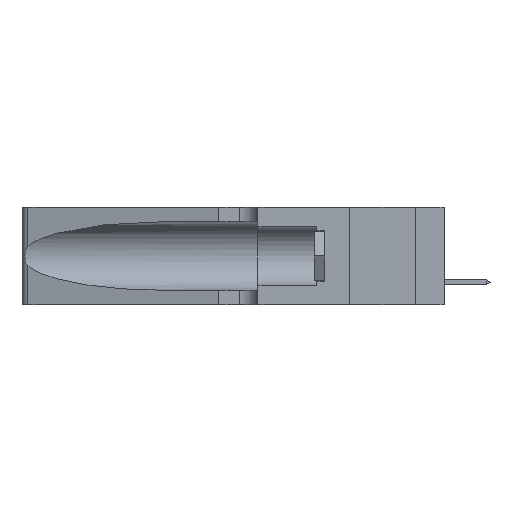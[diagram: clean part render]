
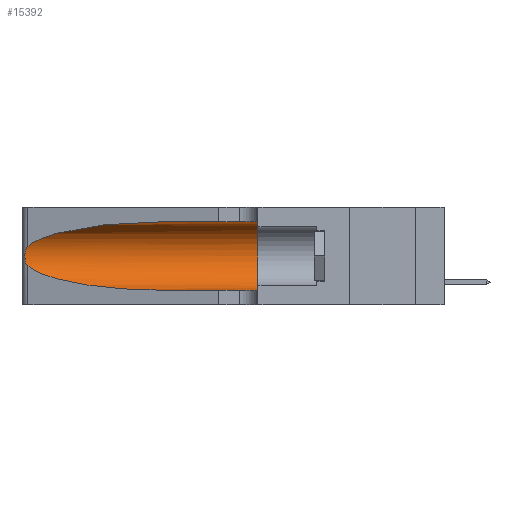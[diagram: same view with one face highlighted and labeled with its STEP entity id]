
A CAD part, left-side view. The second image highlights one B-rep face of the part: STEP entity #15392.
In plain terms, the highlighted cylindrical face has radius 3.308 mm (diameter 6.617 mm), a partial arc.
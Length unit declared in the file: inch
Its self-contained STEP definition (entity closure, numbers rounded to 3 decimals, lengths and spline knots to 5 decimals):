
#442 = EDGE_CURVE ( 'NONE', #17372, #2219, #3135, .T. ) ;
#567 = CARTESIAN_POINT ( 'NONE',  ( 0.26017, 1.23833, 0.17102 ) ) ;
#684 = DIRECTION ( 'NONE',  ( 0., -1., 0. ) ) ;
#1169 = LINE ( 'NONE', #15823, #13541 ) ;
#1185 = DIRECTION ( 'NONE',  ( 0., 1., 0. ) ) ;
#1220 = EDGE_CURVE ( 'NONE', #7691, #2219, #16147, .T. ) ;
#1266 = DIRECTION ( 'NONE',  ( 0., 0., -1. ) ) ;
#1465 = CARTESIAN_POINT ( 'NONE',  ( 0.18966, 0.96281, 0.05475 ) ) ;
#1614 = EDGE_CURVE ( 'NONE', #13062, #11561, #14338, .T. ) ;
#1767 = ORIENTED_EDGE ( 'NONE', *, *, #1220, .T. ) ;
#2219 = VERTEX_POINT ( 'NONE', #5747 ) ;
#2413 = CARTESIAN_POINT ( 'NONE',  ( 0.1305, 0.72297, 0.05475 ) ) ;
#2614 = CARTESIAN_POINT ( 'NONE',  ( 0.1305, 0.35, 0.185 ) ) ;
#3135 = CIRCLE ( 'NONE', #15075, 0.13025 ) ;
#3391 = CARTESIAN_POINT ( 'NONE',  ( 0.26075, 1.23896, 0.19203 ) ) ;
#3633 = CARTESIAN_POINT ( 'NONE',  ( 0.1305, 0.72297, 0.05475 ) ) ;
#4206 = CARTESIAN_POINT ( 'NONE',  ( 0.25487, 1.22718, 0.14631 ) ) ;
#4277 = CARTESIAN_POINT ( 'NONE',  ( 0.1305, 0.72297, 0.31525 ) ) ;
#4448 =( BOUNDED_CURVE ( )  B_SPLINE_CURVE ( 3, ( #14087, #8386, #5746, #15411 ),
 .UNSPECIFIED., .F., .F. ) 
 B_SPLINE_CURVE_WITH_KNOTS ( ( 4, 4 ),
 ( 1.5708, 2.84003 ),
 .UNSPECIFIED. ) 
 CURVE ( )  GEOMETRIC_REPRESENTATION_ITEM ( )  RATIONAL_B_SPLINE_CURVE ( ( 1., 0.87, 0.87, 1. ) ) 
 REPRESENTATION_ITEM ( '' )  );
#4646 = EDGE_CURVE ( 'NONE', #10492, #13062, #4448, .T. ) ;
#4760 = CARTESIAN_POINT ( 'NONE',  ( 0.25487, 1.22718, 0.14631 ) ) ;
#4889 = ORIENTED_EDGE ( 'NONE', *, *, #1614, .T. ) ;
#4906 = CARTESIAN_POINT ( 'NONE',  ( 0.25555, 1.22994, 0.2215 ) ) ;
#5062 = VECTOR ( 'NONE', #5111, 39.37008 ) ;
#5111 = DIRECTION ( 'NONE',  ( 0., -1., 0. ) ) ;
#5331 = DIRECTION ( 'NONE',  ( 0., -1., 0. ) ) ;
#5746 = CARTESIAN_POINT ( 'NONE',  ( 0.2373, 1.15595, 0.28018 ) ) ;
#5747 = CARTESIAN_POINT ( 'NONE',  ( 0.1305, 0.35, 0.05475 ) ) ;
#5951 = EDGE_LOOP ( 'NONE', ( #15759, #4889, #10830, #1767, #12517, #6734 ) ) ;
#6129 = CARTESIAN_POINT ( 'NONE',  ( 0.25856, 1.23593, 0.16098 ) ) ;
#6188 = CARTESIAN_POINT ( 'NONE',  ( 0.26075, 1.23896, 0.178 ) ) ;
#6292 = CARTESIAN_POINT ( 'NONE',  ( 0.25555, 1.22993, 0.14849 ) ) ;
#6547 =( BOUNDED_CURVE ( )  B_SPLINE_CURVE ( 3, ( #4206, #6991, #1465, #2413 ),
 .UNSPECIFIED., .F., .F. ) 
 B_SPLINE_CURVE_WITH_KNOTS ( ( 4, 4 ),
 ( 3.44316, 4.71239 ),
 .UNSPECIFIED. ) 
 CURVE ( )  GEOMETRIC_REPRESENTATION_ITEM ( )  RATIONAL_B_SPLINE_CURVE ( ( 1., 0.87, 0.87, 1. ) ) 
 REPRESENTATION_ITEM ( '' )  );
#6734 = ORIENTED_EDGE ( 'NONE', *, *, #15949, .F. ) ;
#6991 = CARTESIAN_POINT ( 'NONE',  ( 0.2373, 1.15595, 0.08982 ) ) ;
#7266 = FACE_OUTER_BOUND ( 'NONE', #5951, .T. ) ;
#7455 = CARTESIAN_POINT ( 'NONE',  ( 0.25854, 1.2359, 0.20912 ) ) ;
#7691 = VERTEX_POINT ( 'NONE', #3633 ) ;
#8386 = CARTESIAN_POINT ( 'NONE',  ( 0.18966, 0.96281, 0.31525 ) ) ;
#8954 = CARTESIAN_POINT ( 'NONE',  ( 0.25789, 1.23486, 0.15765 ) ) ;
#9500 = DIRECTION ( 'NONE',  ( 0., 0., 1. ) ) ;
#9523 = CARTESIAN_POINT ( 'NONE',  ( 0.1305, 1.61858, 0.185 ) ) ;
#10270 = CYLINDRICAL_SURFACE ( 'NONE', #12976, 0.13025 ) ;
#10342 = CARTESIAN_POINT ( 'NONE',  ( 0.25639, 1.23186, 0.15144 ) ) ;
#10396 = CARTESIAN_POINT ( 'NONE',  ( 0.25487, 1.22718, 0.22369 ) ) ;
#10492 = VERTEX_POINT ( 'NONE', #4277 ) ;
#10830 = ORIENTED_EDGE ( 'NONE', *, *, #15710, .T. ) ;
#11561 = VERTEX_POINT ( 'NONE', #4760 ) ;
#11693 = CARTESIAN_POINT ( 'NONE',  ( 0.25639, 1.23184, 0.21858 ) ) ;
#12120 = CARTESIAN_POINT ( 'NONE',  ( 0.25487, 1.22718, 0.22369 ) ) ;
#12517 = ORIENTED_EDGE ( 'NONE', *, *, #442, .F. ) ;
#12976 = AXIS2_PLACEMENT_3D ( 'NONE', #9523, #5331, #1266 ) ;
#13062 = VERTEX_POINT ( 'NONE', #12120 ) ;
#13063 = CARTESIAN_POINT ( 'NONE',  ( 0.25787, 1.23484, 0.2124 ) ) ;
#13541 = VECTOR ( 'NONE', #684, 39.37008 ) ;
#14087 = CARTESIAN_POINT ( 'NONE',  ( 0.1305, 0.72297, 0.31525 ) ) ;
#14338 = B_SPLINE_CURVE_WITH_KNOTS ( 'NONE', 3,
 ( #10396, #4906, #11693, #13063, #7455, #14602, #3391, #6188, #567, #6129, #8954, #10342, #6292, #15995 ),
 .UNSPECIFIED., .F., .F.,
 ( 4, 2, 2, 2, 2, 2, 4 ),
 ( 0., 0.00027, 0.00053, 0.00107, 0.0016, 0.00187, 0.00214 ),
 .UNSPECIFIED. ) ;
#14398 = CARTESIAN_POINT ( 'NONE',  ( 0.1305, 1.61858, 0.05475 ) ) ;
#14602 = CARTESIAN_POINT ( 'NONE',  ( 0.26018, 1.23835, 0.19895 ) ) ;
#15075 = AXIS2_PLACEMENT_3D ( 'NONE', #2614, #1185, #9500 ) ;
#15392 = ADVANCED_FACE ( 'NONE', ( #7266 ), #10270, .F. ) ;
#15411 = CARTESIAN_POINT ( 'NONE',  ( 0.25487, 1.22718, 0.22369 ) ) ;
#15710 = EDGE_CURVE ( 'NONE', #11561, #7691, #6547, .T. ) ;
#15759 = ORIENTED_EDGE ( 'NONE', *, *, #4646, .T. ) ;
#15823 = CARTESIAN_POINT ( 'NONE',  ( 0.1305, 1.61858, 0.31525 ) ) ;
#15949 = EDGE_CURVE ( 'NONE', #10492, #17372, #1169, .T. ) ;
#15995 = CARTESIAN_POINT ( 'NONE',  ( 0.25487, 1.22718, 0.14631 ) ) ;
#16147 = LINE ( 'NONE', #14398, #5062 ) ;
#16827 = CARTESIAN_POINT ( 'NONE',  ( 0.1305, 0.35, 0.31525 ) ) ;
#17372 = VERTEX_POINT ( 'NONE', #16827 ) ;
